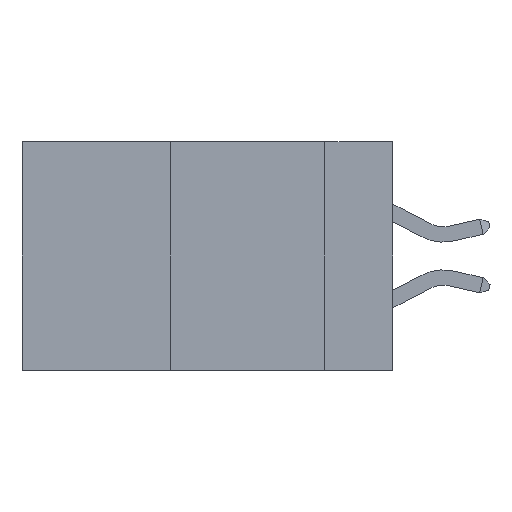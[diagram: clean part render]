
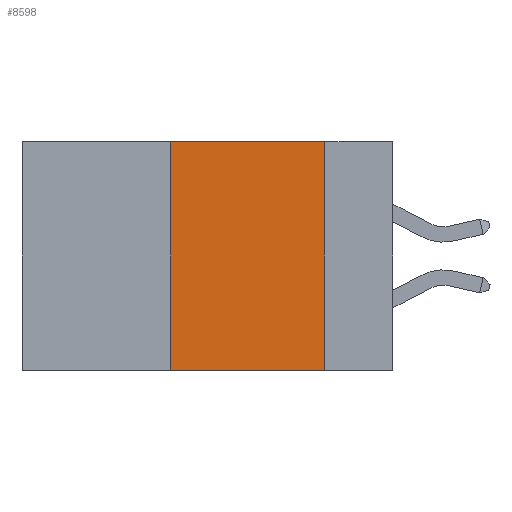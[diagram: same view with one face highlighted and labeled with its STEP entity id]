
A CAD part, left-side view. The second image highlights one B-rep face of the part: STEP entity #8598.
In plain terms, the highlighted planar face has unit normal (-1, 0, 0).
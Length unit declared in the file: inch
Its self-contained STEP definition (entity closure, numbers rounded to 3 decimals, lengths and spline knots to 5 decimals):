
#693 = VECTOR ( 'NONE', #11329, 39.37008 ) ;
#1115 = CARTESIAN_POINT ( 'NONE',  ( 0., 0.6, 0. ) ) ;
#1239 = ORIENTED_EDGE ( 'NONE', *, *, #18033, .F. ) ;
#3868 = LINE ( 'NONE', #23152, #22978 ) ;
#3897 = LINE ( 'NONE', #21252, #26823 ) ;
#5292 = AXIS2_PLACEMENT_3D ( 'NONE', #1115, #5602, #7649 ) ;
#5529 = FACE_OUTER_BOUND ( 'NONE', #26180, .T. ) ;
#5602 = DIRECTION ( 'NONE',  ( 1., 0., 0. ) ) ;
#7335 = LINE ( 'NONE', #13264, #693 ) ;
#7649 = DIRECTION ( 'NONE',  ( 0., 0., -1. ) ) ;
#8598 = ADVANCED_FACE ( 'NONE', ( #5529 ), #27991, .F. ) ;
#11199 = LINE ( 'NONE', #13091, #22991 ) ;
#11329 = DIRECTION ( 'NONE',  ( 0., -1., 0. ) ) ;
#13091 = CARTESIAN_POINT ( 'NONE',  ( 0., 0.36, 0. ) ) ;
#13264 = CARTESIAN_POINT ( 'NONE',  ( 0., 0.6, 0. ) ) ;
#13499 = ORIENTED_EDGE ( 'NONE', *, *, #16428, .F. ) ;
#15257 = VERTEX_POINT ( 'NONE', #25910 ) ;
#15898 = EDGE_CURVE ( 'NONE', #27632, #26634, #3897, .T. ) ;
#16428 = EDGE_CURVE ( 'NONE', #15257, #26634, #3868, .T. ) ;
#16472 = DIRECTION ( 'NONE',  ( 0., 0., -1. ) ) ;
#18033 = EDGE_CURVE ( 'NONE', #27632, #21523, #11199, .T. ) ;
#20431 = ORIENTED_EDGE ( 'NONE', *, *, #28141, .F. ) ;
#21252 = CARTESIAN_POINT ( 'NONE',  ( 0., 0.6, -0.37 ) ) ;
#21523 = VERTEX_POINT ( 'NONE', #22208 ) ;
#21539 = DIRECTION ( 'NONE',  ( 0., 0., 1. ) ) ;
#21547 = DIRECTION ( 'NONE',  ( 0., -1., 0. ) ) ;
#22208 = CARTESIAN_POINT ( 'NONE',  ( 0., 0.36, 0. ) ) ;
#22978 = VECTOR ( 'NONE', #16472, 39.37008 ) ;
#22991 = VECTOR ( 'NONE', #21539, 39.37008 ) ;
#23152 = CARTESIAN_POINT ( 'NONE',  ( 0., 0.11, 0. ) ) ;
#23915 = CARTESIAN_POINT ( 'NONE',  ( 0., 0.36, -0.37 ) ) ;
#25330 = CARTESIAN_POINT ( 'NONE',  ( 0., 0.11, -0.37 ) ) ;
#25675 = ORIENTED_EDGE ( 'NONE', *, *, #15898, .T. ) ;
#25910 = CARTESIAN_POINT ( 'NONE',  ( 0., 0.11, 0. ) ) ;
#26180 = EDGE_LOOP ( 'NONE', ( #13499, #20431, #1239, #25675 ) ) ;
#26634 = VERTEX_POINT ( 'NONE', #25330 ) ;
#26823 = VECTOR ( 'NONE', #21547, 39.37008 ) ;
#27632 = VERTEX_POINT ( 'NONE', #23915 ) ;
#27991 = PLANE ( 'NONE',  #5292 ) ;
#28141 = EDGE_CURVE ( 'NONE', #21523, #15257, #7335, .T. ) ;
